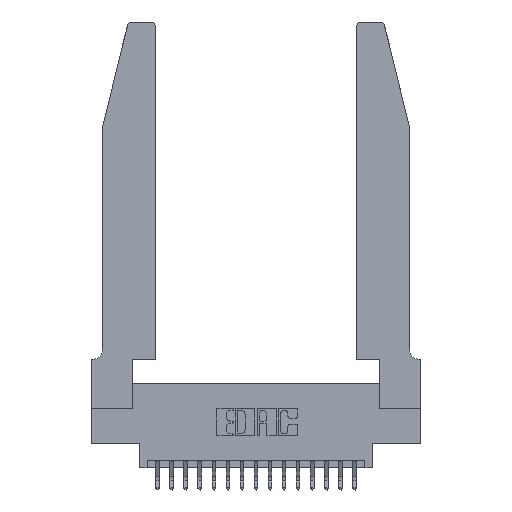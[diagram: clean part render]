
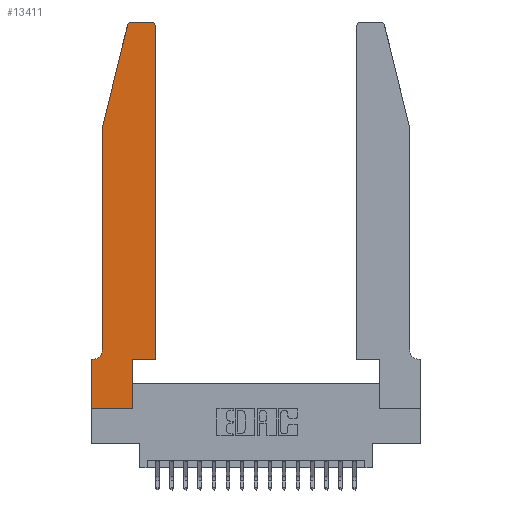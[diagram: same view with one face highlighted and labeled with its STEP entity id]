
A CAD part, top view. The second image highlights one B-rep face of the part: STEP entity #13411.
In plain terms, the highlighted planar face has unit normal (0, 0, 1).
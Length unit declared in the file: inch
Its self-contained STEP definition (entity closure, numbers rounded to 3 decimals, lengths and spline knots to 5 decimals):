
#262 = EDGE_CURVE ( 'NONE', #16669, #15830, #18663, .T. ) ;
#313 = DIRECTION ( 'NONE',  ( 0., -1., 0. ) ) ;
#485 = VERTEX_POINT ( 'NONE', #8370 ) ;
#611 = FACE_OUTER_BOUND ( 'NONE', #18463, .T. ) ;
#675 = CARTESIAN_POINT ( 'NONE',  ( 0.0755, 2., 0.37 ) ) ;
#734 = CIRCLE ( 'NONE', #5775, 0.03 ) ;
#810 = EDGE_CURVE ( 'NONE', #5051, #1135, #17406, .T. ) ;
#887 = ORIENTED_EDGE ( 'NONE', *, *, #4227, .T. ) ;
#1098 = CARTESIAN_POINT ( 'NONE',  ( 0.25487, 2.72718, 0.37 ) ) ;
#1135 = VERTEX_POINT ( 'NONE', #14052 ) ;
#1267 = EDGE_CURVE ( 'NONE', #10910, #15642, #18538, .T. ) ;
#1400 = LINE ( 'NONE', #9878, #8866 ) ;
#1549 = EDGE_CURVE ( 'NONE', #17558, #485, #19255, .T. ) ;
#1708 = ORIENTED_EDGE ( 'NONE', *, *, #12577, .T. ) ;
#1769 = DIRECTION ( 'NONE',  ( 0., 0., -1. ) ) ;
#2614 = CARTESIAN_POINT ( 'NONE',  ( 0.0755, 2., 0.37 ) ) ;
#2829 = EDGE_CURVE ( 'NONE', #15642, #16669, #10483, .T. ) ;
#3471 = ORIENTED_EDGE ( 'NONE', *, *, #14481, .T. ) ;
#3845 = VERTEX_POINT ( 'NONE', #14203 ) ;
#4182 = CARTESIAN_POINT ( 'NONE',  ( 0.284, 2.72, 0.37 ) ) ;
#4227 = EDGE_CURVE ( 'NONE', #15830, #5051, #12946, .T. ) ;
#4455 = CARTESIAN_POINT ( 'NONE',  ( 0.0755, 0.42, 0.37 ) ) ;
#4653 = DIRECTION ( 'NONE',  ( 0., 0., 1. ) ) ;
#4671 = DIRECTION ( 'NONE',  ( 0., 0., 1. ) ) ;
#4758 = DIRECTION ( 'NONE',  ( 0., 1., 0. ) ) ;
#4870 = VERTEX_POINT ( 'NONE', #8209 ) ;
#5051 = VERTEX_POINT ( 'NONE', #11729 ) ;
#5204 = CARTESIAN_POINT ( 'NONE',  ( 0.0055, 0.42, 0.37 ) ) ;
#5775 = AXIS2_PLACEMENT_3D ( 'NONE', #17064, #4671, #7842 ) ;
#5844 = ORIENTED_EDGE ( 'NONE', *, *, #262, .T. ) ;
#6167 = ORIENTED_EDGE ( 'NONE', *, *, #2829, .T. ) ;
#6403 = ORIENTED_EDGE ( 'NONE', *, *, #1549, .T. ) ;
#6724 = DIRECTION ( 'NONE',  ( -1., 0., 0. ) ) ;
#6742 = VECTOR ( 'NONE', #313, 39.37008 ) ;
#7151 = CARTESIAN_POINT ( 'NONE',  ( 0.2865, 0.35, 0.37 ) ) ;
#7374 = DIRECTION ( 'NONE',  ( 0., 0., 1. ) ) ;
#7420 = EDGE_CURVE ( 'NONE', #13287, #20164, #11852, .T. ) ;
#7614 = VECTOR ( 'NONE', #12938, 39.37008 ) ;
#7639 = VECTOR ( 'NONE', #13333, 39.37008 ) ;
#7842 = DIRECTION ( 'NONE',  ( 1., 0., 0. ) ) ;
#7963 = ORIENTED_EDGE ( 'NONE', *, *, #1267, .T. ) ;
#8019 = DIRECTION ( 'NONE',  ( -1., 0., 0. ) ) ;
#8209 = CARTESIAN_POINT ( 'NONE',  ( 0.4205, 2.75, 0.37 ) ) ;
#8370 = CARTESIAN_POINT ( 'NONE',  ( 0.4505, 2.72, 0.37 ) ) ;
#8866 = VECTOR ( 'NONE', #14689, 39.37008 ) ;
#8964 = ORIENTED_EDGE ( 'NONE', *, *, #16334, .T. ) ;
#8974 = ORIENTED_EDGE ( 'NONE', *, *, #810, .T. ) ;
#9146 = DIRECTION ( 'NONE',  ( 0., -1., 0. ) ) ;
#9301 = CARTESIAN_POINT ( 'NONE',  ( 0., 0., 0.37 ) ) ;
#9609 = DIRECTION ( 'NONE',  ( 1., 0., 0. ) ) ;
#9687 = VECTOR ( 'NONE', #8019, 39.37008 ) ;
#9814 = AXIS2_PLACEMENT_3D ( 'NONE', #4182, #7374, #10683 ) ;
#9827 = CARTESIAN_POINT ( 'NONE',  ( 0., 0., 0.37 ) ) ;
#9878 = CARTESIAN_POINT ( 'NONE',  ( 0.2605, 2.75, 0.37 ) ) ;
#10483 = LINE ( 'NONE', #675, #19923 ) ;
#10528 = VECTOR ( 'NONE', #20369, 39.37008 ) ;
#10683 = DIRECTION ( 'NONE',  ( 1., 0., 0. ) ) ;
#10840 = CARTESIAN_POINT ( 'NONE',  ( 0.4505, 0.35, 0.37 ) ) ;
#10910 = VERTEX_POINT ( 'NONE', #1098 ) ;
#10940 = EDGE_CURVE ( 'NONE', #485, #4870, #734, .T. ) ;
#11552 = LINE ( 'NONE', #9301, #10528 ) ;
#11729 = CARTESIAN_POINT ( 'NONE',  ( 0., 0.35, 0.37 ) ) ;
#11792 = EDGE_CURVE ( 'NONE', #20164, #17558, #13059, .T. ) ;
#11852 = LINE ( 'NONE', #7151, #7639 ) ;
#12577 = EDGE_CURVE ( 'NONE', #1135, #13287, #11552, .T. ) ;
#12938 = DIRECTION ( 'NONE',  ( -0.239, -0.971, 0. ) ) ;
#12946 = LINE ( 'NONE', #15833, #9687 ) ;
#12983 = AXIS2_PLACEMENT_3D ( 'NONE', #15707, #4653, #9609 ) ;
#13059 = LINE ( 'NONE', #16891, #20232 ) ;
#13287 = VERTEX_POINT ( 'NONE', #19771 ) ;
#13333 = DIRECTION ( 'NONE',  ( 0., 1., 0. ) ) ;
#13411 = ADVANCED_FACE ( 'NONE', ( #611 ), #17387, .T. ) ;
#13889 = ORIENTED_EDGE ( 'NONE', *, *, #10940, .T. ) ;
#14052 = CARTESIAN_POINT ( 'NONE',  ( 0., 0., 0.37 ) ) ;
#14187 = CARTESIAN_POINT ( 'NONE',  ( 0.4505, 0.35, 0.37 ) ) ;
#14203 = CARTESIAN_POINT ( 'NONE',  ( 0.284, 2.75, 0.37 ) ) ;
#14481 = EDGE_CURVE ( 'NONE', #4870, #3845, #1400, .T. ) ;
#14689 = DIRECTION ( 'NONE',  ( -1., 0., 0. ) ) ;
#15477 = ORIENTED_EDGE ( 'NONE', *, *, #7420, .T. ) ;
#15642 = VERTEX_POINT ( 'NONE', #2614 ) ;
#15707 = CARTESIAN_POINT ( 'NONE',  ( 0., 0.35, 0.37 ) ) ;
#15830 = VERTEX_POINT ( 'NONE', #16497 ) ;
#15833 = CARTESIAN_POINT ( 'NONE',  ( 0.0755, 0.35, 0.37 ) ) ;
#16314 = CARTESIAN_POINT ( 'NONE',  ( 0.2865, 0.35, 0.37 ) ) ;
#16334 = EDGE_CURVE ( 'NONE', #3845, #10910, #18924, .T. ) ;
#16497 = CARTESIAN_POINT ( 'NONE',  ( 0.0055, 0.35, 0.37 ) ) ;
#16669 = VERTEX_POINT ( 'NONE', #4455 ) ;
#16891 = CARTESIAN_POINT ( 'NONE',  ( 0.4505, 0.35, 0.37 ) ) ;
#16958 = DIRECTION ( 'NONE',  ( 1., 0., 0. ) ) ;
#17064 = CARTESIAN_POINT ( 'NONE',  ( 0.4205, 2.72, 0.37 ) ) ;
#17348 = ORIENTED_EDGE ( 'NONE', *, *, #11792, .T. ) ;
#17387 = PLANE ( 'NONE',  #12983 ) ;
#17406 = LINE ( 'NONE', #9827, #6742 ) ;
#17558 = VERTEX_POINT ( 'NONE', #14187 ) ;
#18016 = VECTOR ( 'NONE', #4758, 39.37008 ) ;
#18463 = EDGE_LOOP ( 'NONE', ( #3471, #8964, #7963, #6167, #5844, #887, #8974, #1708, #15477, #17348, #6403, #13889 ) ) ;
#18538 = LINE ( 'NONE', #19173, #7614 ) ;
#18663 = CIRCLE ( 'NONE', #19056, 0.07 ) ;
#18924 = CIRCLE ( 'NONE', #9814, 0.03 ) ;
#19056 = AXIS2_PLACEMENT_3D ( 'NONE', #5204, #1769, #6724 ) ;
#19173 = CARTESIAN_POINT ( 'NONE',  ( 0.0755, 2., 0.37 ) ) ;
#19255 = LINE ( 'NONE', #10840, #18016 ) ;
#19771 = CARTESIAN_POINT ( 'NONE',  ( 0.2865, 0., 0.37 ) ) ;
#19923 = VECTOR ( 'NONE', #9146, 39.37008 ) ;
#20164 = VERTEX_POINT ( 'NONE', #16314 ) ;
#20232 = VECTOR ( 'NONE', #16958, 39.37008 ) ;
#20369 = DIRECTION ( 'NONE',  ( 1., 0., 0. ) ) ;
